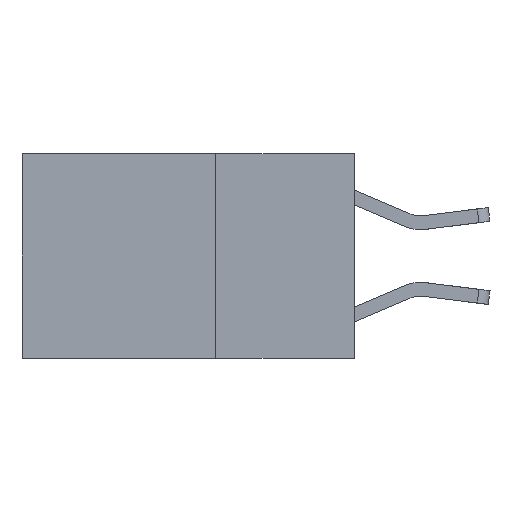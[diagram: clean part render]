
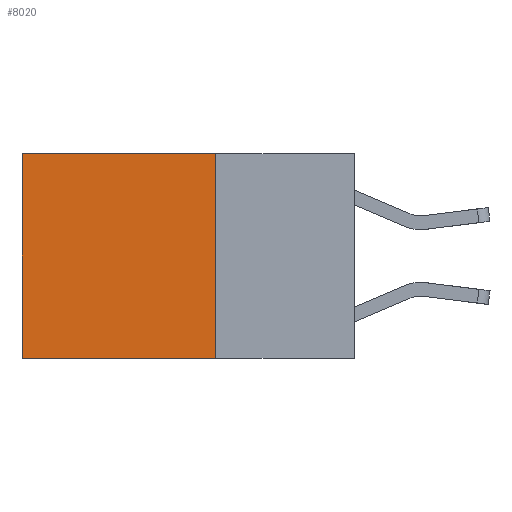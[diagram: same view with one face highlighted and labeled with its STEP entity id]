
A CAD part, left-side view. The second image highlights one B-rep face of the part: STEP entity #8020.
In plain terms, the highlighted planar face has unit normal (-1, 0, 0).
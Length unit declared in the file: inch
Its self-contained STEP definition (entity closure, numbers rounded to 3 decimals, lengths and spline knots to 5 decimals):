
#343 = VERTEX_POINT ( 'NONE', #1269 ) ;
#374 = FACE_OUTER_BOUND ( 'NONE', #4189, .T. ) ;
#579 = CARTESIAN_POINT ( 'NONE',  ( 0.2625, 0.25, -0.37 ) ) ;
#702 = DIRECTION ( 'NONE',  ( 1., 0., 0. ) ) ;
#1269 = CARTESIAN_POINT ( 'NONE',  ( 0.2625, 0.25, -0.37 ) ) ;
#1850 = CARTESIAN_POINT ( 'NONE',  ( 0.2625, 0.6, 0. ) ) ;
#2880 = VECTOR ( 'NONE', #7952, 39.37008 ) ;
#3142 = DIRECTION ( 'NONE',  ( 0., 1., 0. ) ) ;
#3274 = VECTOR ( 'NONE', #3142, 39.37008 ) ;
#3298 = CARTESIAN_POINT ( 'NONE',  ( 0.2625, 0.25, 0. ) ) ;
#4189 = EDGE_LOOP ( 'NONE', ( #8459, #7550, #7675, #7660 ) ) ;
#4249 = VECTOR ( 'NONE', #6784, 39.37008 ) ;
#4773 = LINE ( 'NONE', #9192, #6975 ) ;
#5221 = AXIS2_PLACEMENT_3D ( 'NONE', #3298, #702, #6898 ) ;
#5539 = VERTEX_POINT ( 'NONE', #7882 ) ;
#5666 = DIRECTION ( 'NONE',  ( 0., 0., -1. ) ) ;
#5706 = VERTEX_POINT ( 'NONE', #10534 ) ;
#5868 = EDGE_CURVE ( 'NONE', #343, #10991, #10863, .T. ) ;
#6685 = EDGE_CURVE ( 'NONE', #5706, #343, #4773, .T. ) ;
#6784 = DIRECTION ( 'NONE',  ( 0., 1., 0. ) ) ;
#6898 = DIRECTION ( 'NONE',  ( 0., 0., -1. ) ) ;
#6975 = VECTOR ( 'NONE', #5666, 39.37008 ) ;
#7550 = ORIENTED_EDGE ( 'NONE', *, *, #5868, .F. ) ;
#7660 = ORIENTED_EDGE ( 'NONE', *, *, #8362, .T. ) ;
#7675 = ORIENTED_EDGE ( 'NONE', *, *, #6685, .F. ) ;
#7736 = LINE ( 'NONE', #10858, #3274 ) ;
#7882 = CARTESIAN_POINT ( 'NONE',  ( 0.2625, 0.6, 0. ) ) ;
#7952 = DIRECTION ( 'NONE',  ( 0., 0., -1. ) ) ;
#8020 = ADVANCED_FACE ( 'NONE', ( #374 ), #10996, .F. ) ;
#8362 = EDGE_CURVE ( 'NONE', #5706, #5539, #7736, .T. ) ;
#8459 = ORIENTED_EDGE ( 'NONE', *, *, #8496, .T. ) ;
#8496 = EDGE_CURVE ( 'NONE', #5539, #10991, #9564, .T. ) ;
#9192 = CARTESIAN_POINT ( 'NONE',  ( 0.2625, 0.25, 0. ) ) ;
#9564 = LINE ( 'NONE', #1850, #2880 ) ;
#10534 = CARTESIAN_POINT ( 'NONE',  ( 0.2625, 0.25, 0. ) ) ;
#10858 = CARTESIAN_POINT ( 'NONE',  ( 0.2625, 0.25, 0. ) ) ;
#10863 = LINE ( 'NONE', #579, #4249 ) ;
#10991 = VERTEX_POINT ( 'NONE', #11022 ) ;
#10996 = PLANE ( 'NONE',  #5221 ) ;
#11022 = CARTESIAN_POINT ( 'NONE',  ( 0.2625, 0.6, -0.37 ) ) ;
